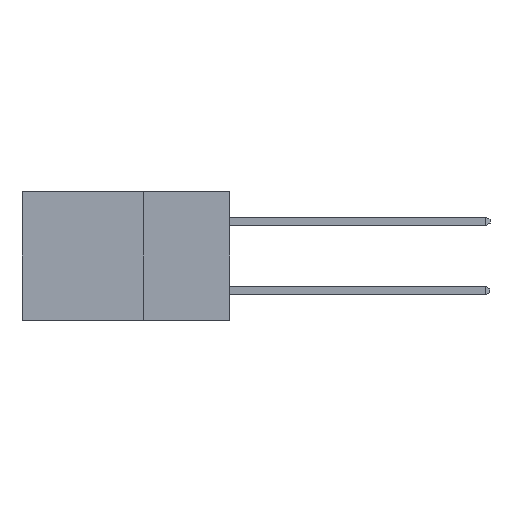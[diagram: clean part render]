
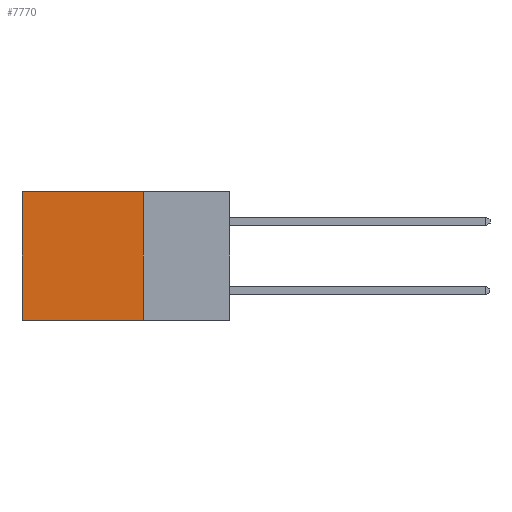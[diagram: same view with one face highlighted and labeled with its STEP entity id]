
A CAD part, left-side view. The second image highlights one B-rep face of the part: STEP entity #7770.
In plain terms, the highlighted planar face has unit normal (-1, 0, 0).
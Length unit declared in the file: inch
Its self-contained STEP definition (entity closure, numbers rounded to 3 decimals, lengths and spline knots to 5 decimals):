
#53 = CARTESIAN_POINT ( 'NONE',  ( 0.298, 0.25, -0.37 ) ) ;
#1206 = VECTOR ( 'NONE', #18140, 39.37008 ) ;
#2750 = CARTESIAN_POINT ( 'NONE',  ( 0.298, 0.25, 0. ) ) ;
#2765 = VECTOR ( 'NONE', #24422, 39.37008 ) ;
#3627 = VECTOR ( 'NONE', #20878, 39.37008 ) ;
#3679 = VECTOR ( 'NONE', #23095, 39.37008 ) ;
#3986 = VERTEX_POINT ( 'NONE', #4552 ) ;
#4149 = CARTESIAN_POINT ( 'NONE',  ( 0.298, 0.25, 0. ) ) ;
#4552 = CARTESIAN_POINT ( 'NONE',  ( 0.298, 0.25, -0.37 ) ) ;
#4915 = LINE ( 'NONE', #53, #3679 ) ;
#5580 = CARTESIAN_POINT ( 'NONE',  ( 0.298, 0.6, 0. ) ) ;
#7770 = ADVANCED_FACE ( 'NONE', ( #10502 ), #20203, .F. ) ;
#8728 = LINE ( 'NONE', #5580, #3627 ) ;
#9453 = ORIENTED_EDGE ( 'NONE', *, *, #22797, .T. ) ;
#10502 = FACE_OUTER_BOUND ( 'NONE', #23223, .T. ) ;
#10646 = DIRECTION ( 'NONE',  ( 0., 0., -1. ) ) ;
#12085 = LINE ( 'NONE', #2750, #1206 ) ;
#12482 = ORIENTED_EDGE ( 'NONE', *, *, #18793, .F. ) ;
#13645 = LINE ( 'NONE', #22594, #2765 ) ;
#13780 = AXIS2_PLACEMENT_3D ( 'NONE', #14514, #22102, #10646 ) ;
#13911 = EDGE_CURVE ( 'NONE', #24352, #24220, #13645, .T. ) ;
#14514 = CARTESIAN_POINT ( 'NONE',  ( 0.298, 0.25, 0. ) ) ;
#15994 = ORIENTED_EDGE ( 'NONE', *, *, #13911, .T. ) ;
#16159 = CARTESIAN_POINT ( 'NONE',  ( 0.298, 0.6, -0.37 ) ) ;
#17181 = CARTESIAN_POINT ( 'NONE',  ( 0.298, 0.6, 0. ) ) ;
#18140 = DIRECTION ( 'NONE',  ( 0., 0., -1. ) ) ;
#18793 = EDGE_CURVE ( 'NONE', #24352, #3986, #12085, .T. ) ;
#19427 = VERTEX_POINT ( 'NONE', #16159 ) ;
#20203 = PLANE ( 'NONE',  #13780 ) ;
#20878 = DIRECTION ( 'NONE',  ( 0., 0., -1. ) ) ;
#21866 = ORIENTED_EDGE ( 'NONE', *, *, #21946, .F. ) ;
#21946 = EDGE_CURVE ( 'NONE', #3986, #19427, #4915, .T. ) ;
#22102 = DIRECTION ( 'NONE',  ( 1., 0., 0. ) ) ;
#22594 = CARTESIAN_POINT ( 'NONE',  ( 0.298, 0.25, 0. ) ) ;
#22797 = EDGE_CURVE ( 'NONE', #24220, #19427, #8728, .T. ) ;
#23095 = DIRECTION ( 'NONE',  ( 0., 1., 0. ) ) ;
#23223 = EDGE_LOOP ( 'NONE', ( #9453, #21866, #12482, #15994 ) ) ;
#24220 = VERTEX_POINT ( 'NONE', #17181 ) ;
#24352 = VERTEX_POINT ( 'NONE', #4149 ) ;
#24422 = DIRECTION ( 'NONE',  ( 0., 1., 0. ) ) ;
